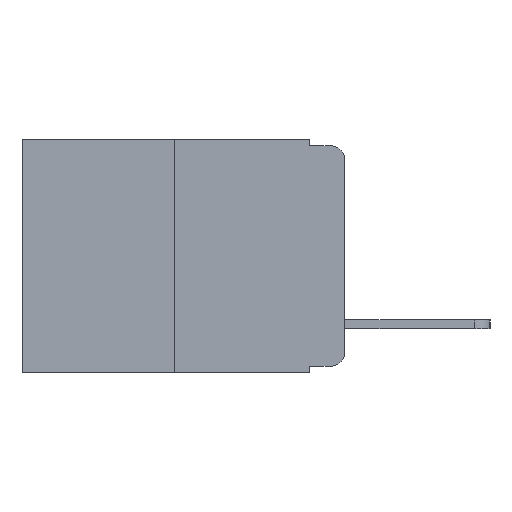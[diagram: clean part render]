
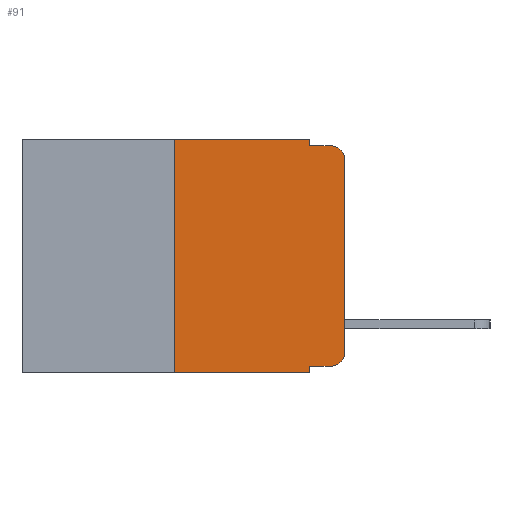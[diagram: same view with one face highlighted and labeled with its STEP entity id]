
A CAD part, left-side view. The second image highlights one B-rep face of the part: STEP entity #91.
In plain terms, the highlighted planar face has unit normal (-1, 0, 0).
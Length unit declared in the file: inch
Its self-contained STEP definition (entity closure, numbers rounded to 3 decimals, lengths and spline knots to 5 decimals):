
#65 = EDGE_LOOP ( 'NONE', ( #3687, #13968, #13441, #12404, #2215, #12397, #9546, #11401, #1889, #2130 ) ) ;
#91 = ADVANCED_FACE ( 'NONE', ( #11809 ), #7259, .F. ) ;
#718 = CARTESIAN_POINT ( 'NONE',  ( 0., 0., -0.313 ) ) ;
#1586 = CARTESIAN_POINT ( 'NONE',  ( 0., 0.051, 0. ) ) ;
#1677 = DIRECTION ( 'NONE',  ( -1., 0., 0. ) ) ;
#1835 = CARTESIAN_POINT ( 'NONE',  ( 0., 0.051, -0.343 ) ) ;
#1861 = CARTESIAN_POINT ( 'NONE',  ( 0., 0.051, -0.333 ) ) ;
#1864 = VERTEX_POINT ( 'NONE', #6748 ) ;
#1889 = ORIENTED_EDGE ( 'NONE', *, *, #12541, .T. ) ;
#2004 = DIRECTION ( 'NONE',  ( 0., 0., -1. ) ) ;
#2130 = ORIENTED_EDGE ( 'NONE', *, *, #8780, .T. ) ;
#2215 = ORIENTED_EDGE ( 'NONE', *, *, #5599, .F. ) ;
#2438 = DIRECTION ( 'NONE',  ( -1., 0., 0. ) ) ;
#2945 = VERTEX_POINT ( 'NONE', #1586 ) ;
#3223 = AXIS2_PLACEMENT_3D ( 'NONE', #8589, #1677, #9769 ) ;
#3243 = DIRECTION ( 'NONE',  ( 0., -1., 0. ) ) ;
#3321 = VERTEX_POINT ( 'NONE', #3535 ) ;
#3389 = CARTESIAN_POINT ( 'NONE',  ( 0., 0.051, -0.01 ) ) ;
#3535 = CARTESIAN_POINT ( 'NONE',  ( 0., 0.25, 0. ) ) ;
#3687 = ORIENTED_EDGE ( 'NONE', *, *, #5013, .T. ) ;
#3898 = CARTESIAN_POINT ( 'NONE',  ( 0., 0.02, -0.01 ) ) ;
#4062 = VECTOR ( 'NONE', #2004, 39.37008 ) ;
#4153 = EDGE_CURVE ( 'NONE', #1864, #3321, #11551, .T. ) ;
#4368 = CARTESIAN_POINT ( 'NONE',  ( 0., 0., 0. ) ) ;
#4499 = EDGE_CURVE ( 'NONE', #12588, #8566, #6450, .T. ) ;
#4520 = CARTESIAN_POINT ( 'NONE',  ( 0., 0., -0.03 ) ) ;
#4632 = VECTOR ( 'NONE', #12453, 39.37008 ) ;
#4812 = CIRCLE ( 'NONE', #10601, 0.02 ) ;
#4831 = LINE ( 'NONE', #10991, #10282 ) ;
#5009 = VECTOR ( 'NONE', #13093, 39.37008 ) ;
#5013 = EDGE_CURVE ( 'NONE', #13839, #12212, #10808, .T. ) ;
#5387 = CARTESIAN_POINT ( 'NONE',  ( 0., 0.051, 0. ) ) ;
#5599 = EDGE_CURVE ( 'NONE', #3321, #2945, #9190, .T. ) ;
#5917 = EDGE_CURVE ( 'NONE', #12212, #8566, #4812, .T. ) ;
#6300 = DIRECTION ( 'NONE',  ( 0., 0., -1. ) ) ;
#6450 = LINE ( 'NONE', #3389, #12609 ) ;
#6748 = CARTESIAN_POINT ( 'NONE',  ( 0., 0.25, -0.343 ) ) ;
#6852 = EDGE_CURVE ( 'NONE', #2945, #12588, #10235, .T. ) ;
#7011 = DIRECTION ( 'NONE',  ( 1., 0., 0. ) ) ;
#7259 = PLANE ( 'NONE',  #8606 ) ;
#8198 = EDGE_CURVE ( 'NONE', #1864, #14793, #12977, .T. ) ;
#8257 = CARTESIAN_POINT ( 'NONE',  ( 0., 0.02, -0.333 ) ) ;
#8474 = CIRCLE ( 'NONE', #3223, 0.02 ) ;
#8566 = VERTEX_POINT ( 'NONE', #3898 ) ;
#8589 = CARTESIAN_POINT ( 'NONE',  ( 0., 0.02, -0.313 ) ) ;
#8606 = AXIS2_PLACEMENT_3D ( 'NONE', #8908, #7011, #8729 ) ;
#8636 = EDGE_CURVE ( 'NONE', #13130, #14793, #4831, .T. ) ;
#8637 = DIRECTION ( 'NONE',  ( 0., -1., 0. ) ) ;
#8729 = DIRECTION ( 'NONE',  ( 0., 0., -1. ) ) ;
#8780 = EDGE_CURVE ( 'NONE', #10382, #13839, #8474, .T. ) ;
#8825 = VECTOR ( 'NONE', #11389, 39.37008 ) ;
#8908 = CARTESIAN_POINT ( 'NONE',  ( 0., 0.473, 0. ) ) ;
#9190 = LINE ( 'NONE', #13705, #8825 ) ;
#9360 = CARTESIAN_POINT ( 'NONE',  ( 0., 0.02, -0.03 ) ) ;
#9546 = ORIENTED_EDGE ( 'NONE', *, *, #8198, .T. ) ;
#9769 = DIRECTION ( 'NONE',  ( 0., 0., -1. ) ) ;
#9905 = CARTESIAN_POINT ( 'NONE',  ( 0., 0.051, -0.01 ) ) ;
#9936 = VECTOR ( 'NONE', #3243, 39.37008 ) ;
#10235 = LINE ( 'NONE', #5387, #4062 ) ;
#10282 = VECTOR ( 'NONE', #6300, 39.37008 ) ;
#10382 = VERTEX_POINT ( 'NONE', #8257 ) ;
#10504 = DIRECTION ( 'NONE',  ( 0., 0., -1. ) ) ;
#10601 = AXIS2_PLACEMENT_3D ( 'NONE', #9360, #2438, #10504 ) ;
#10719 = LINE ( 'NONE', #10959, #13767 ) ;
#10808 = LINE ( 'NONE', #4368, #4632 ) ;
#10959 = CARTESIAN_POINT ( 'NONE',  ( 0., 0.051, -0.333 ) ) ;
#10991 = CARTESIAN_POINT ( 'NONE',  ( 0., 0.051, 0. ) ) ;
#11389 = DIRECTION ( 'NONE',  ( 0., -1., 0. ) ) ;
#11401 = ORIENTED_EDGE ( 'NONE', *, *, #8636, .F. ) ;
#11474 = DIRECTION ( 'NONE',  ( 0., -1., 0. ) ) ;
#11551 = LINE ( 'NONE', #14242, #5009 ) ;
#11809 = FACE_OUTER_BOUND ( 'NONE', #65, .T. ) ;
#12212 = VERTEX_POINT ( 'NONE', #4520 ) ;
#12397 = ORIENTED_EDGE ( 'NONE', *, *, #4153, .F. ) ;
#12404 = ORIENTED_EDGE ( 'NONE', *, *, #6852, .F. ) ;
#12453 = DIRECTION ( 'NONE',  ( 0., 0., 1. ) ) ;
#12541 = EDGE_CURVE ( 'NONE', #13130, #10382, #10719, .T. ) ;
#12588 = VERTEX_POINT ( 'NONE', #9905 ) ;
#12609 = VECTOR ( 'NONE', #11474, 39.37008 ) ;
#12977 = LINE ( 'NONE', #14733, #9936 ) ;
#13093 = DIRECTION ( 'NONE',  ( 0., 0., 1. ) ) ;
#13130 = VERTEX_POINT ( 'NONE', #1861 ) ;
#13441 = ORIENTED_EDGE ( 'NONE', *, *, #4499, .F. ) ;
#13705 = CARTESIAN_POINT ( 'NONE',  ( 0., 0.473, 0. ) ) ;
#13767 = VECTOR ( 'NONE', #8637, 39.37008 ) ;
#13839 = VERTEX_POINT ( 'NONE', #718 ) ;
#13968 = ORIENTED_EDGE ( 'NONE', *, *, #5917, .T. ) ;
#14242 = CARTESIAN_POINT ( 'NONE',  ( 0., 0.25, 0. ) ) ;
#14733 = CARTESIAN_POINT ( 'NONE',  ( 0., 0.473, -0.343 ) ) ;
#14793 = VERTEX_POINT ( 'NONE', #1835 ) ;
